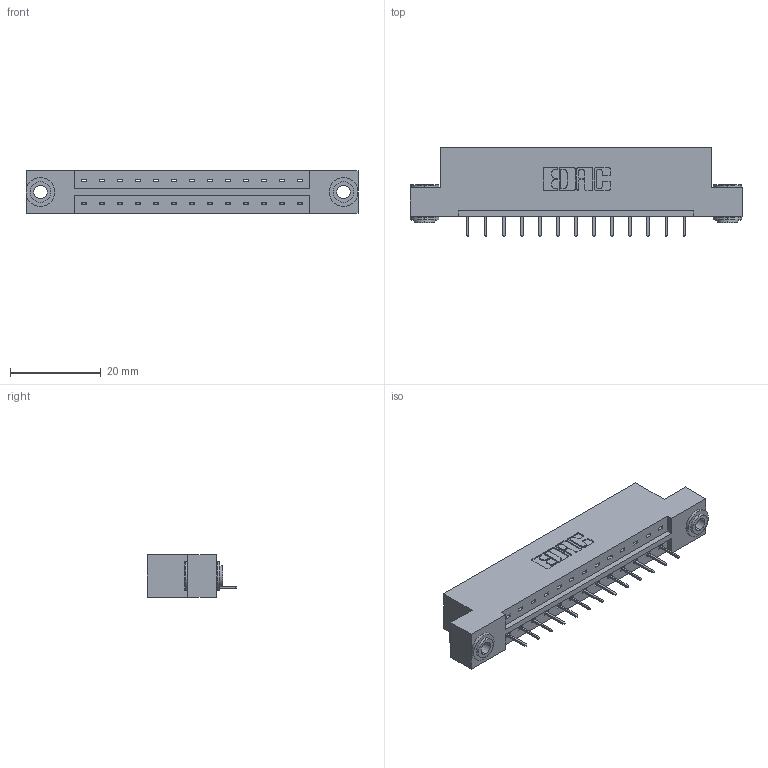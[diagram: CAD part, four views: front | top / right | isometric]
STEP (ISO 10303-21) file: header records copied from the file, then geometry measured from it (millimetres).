
FILE_DESCRIPTION (( 'STEP AP203' ), '1' );
FILE_NAME ('833-013-524-103.STEP', '2020-05-30T23:51:46', ( '' ), ( '' ), 'SwSTEP 2.0', 'SolidWorks 2020', '' );
FILE_SCHEMA (( 'CONFIG_CONTROL_DESIGN' ));
Length unit declared in the file: inch
Products named in the file (4): 345-292-001_345-293-124; 833-013-524-103; 833 Part_Flush - .156 Dia - TH; 345-250-002_345-250-002-102
Assembly tree (16 placements, depth 2):
  833-013-524-103
    833 Part_Flush - .156 Dia - TH
    345-292-001_345-293-124  x13
    345-250-002_345-250-002-102  x2
Bounding box: 73.05 x 19.69 x 9.4 mm (x, y, z)
Volume: 7069.6 mm3; surface area: 7510.4 mm2
Topology: 16 solids, 16 shells, 958 faces, 2727 edges, 1762 vertices
Faces by surface type: plane 704, cylinder 246, cone 8
Entity records: 12422 total; most frequent: CARTESIAN_POINT 2124, ORIENTED_EDGE 2066, DIRECTION 1885, EDGE_CURVE 1033, VECTOR 885, LINE 885, VERTEX_POINT 682, AXIS2_PLACEMENT_3D 500
